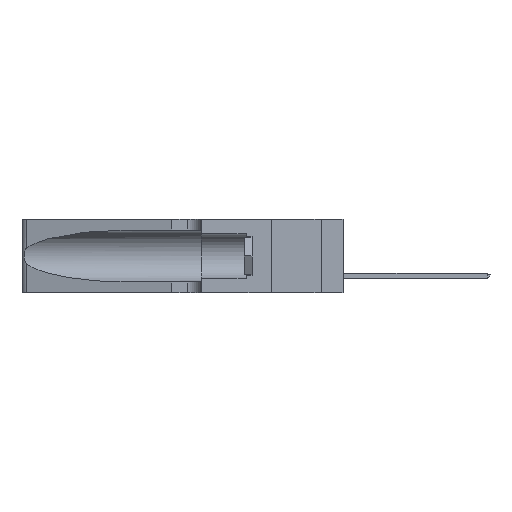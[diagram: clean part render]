
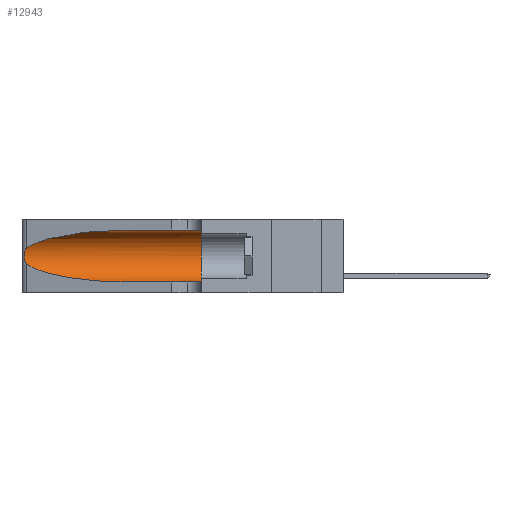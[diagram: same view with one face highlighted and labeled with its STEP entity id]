
A CAD part, left-side view. The second image highlights one B-rep face of the part: STEP entity #12943.
In plain terms, the highlighted cylindrical face has radius 3.308 mm (diameter 6.617 mm), a partial arc.
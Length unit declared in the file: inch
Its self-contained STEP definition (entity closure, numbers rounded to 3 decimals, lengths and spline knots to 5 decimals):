
#659 = LINE ( 'NONE', #36395, #18761 ) ;
#978 = CARTESIAN_POINT ( 'NONE',  ( 0.25487, 1.22718, 0.22369 ) ) ;
#2302 = AXIS2_PLACEMENT_3D ( 'NONE', #22940, #5608, #25963 ) ;
#2400 = VERTEX_POINT ( 'NONE', #12717 ) ;
#2910 = CARTESIAN_POINT ( 'NONE',  ( 0.2373, 1.15595, 0.08982 ) ) ;
#3451 = EDGE_CURVE ( 'NONE', #35282, #16058, #29816, .T. ) ;
#4575 = VERTEX_POINT ( 'NONE', #32277 ) ;
#4591 = ORIENTED_EDGE ( 'NONE', *, *, #21053, .T. ) ;
#4667 = DIRECTION ( 'NONE',  ( 0., 0., -1. ) ) ;
#5193 = EDGE_LOOP ( 'NONE', ( #29478, #30872, #4591, #17342, #19111, #34222 ) ) ;
#5608 = DIRECTION ( 'NONE',  ( 0., 1., 0. ) ) ;
#6177 = CARTESIAN_POINT ( 'NONE',  ( 0.1305, 1.61858, 0.185 ) ) ;
#6301 = CARTESIAN_POINT ( 'NONE',  ( 0.25639, 1.23184, 0.21858 ) ) ;
#6502 = CARTESIAN_POINT ( 'NONE',  ( 0.25487, 1.22718, 0.14631 ) ) ;
#6692 = CARTESIAN_POINT ( 'NONE',  ( 0.25639, 1.23186, 0.15144 ) ) ;
#6892 =( BOUNDED_CURVE ( )  B_SPLINE_CURVE ( 3, ( #6502, #2910, #17912, #18145 ),
 .UNSPECIFIED., .F., .F. ) 
 B_SPLINE_CURVE_WITH_KNOTS ( ( 4, 4 ),
 ( 3.44316, 4.71239 ),
 .UNSPECIFIED. ) 
 CURVE ( )  GEOMETRIC_REPRESENTATION_ITEM ( )  RATIONAL_B_SPLINE_CURVE ( ( 1., 0.87, 0.87, 1. ) ) 
 REPRESENTATION_ITEM ( '' )  );
#7672 = CARTESIAN_POINT ( 'NONE',  ( 0.25487, 1.22718, 0.22369 ) ) ;
#8456 = CIRCLE ( 'NONE', #2302, 0.13025 ) ;
#9170 = CARTESIAN_POINT ( 'NONE',  ( 0.18966, 0.96281, 0.31525 ) ) ;
#9210 = EDGE_CURVE ( 'NONE', #4575, #32043, #659, .T. ) ;
#9219 = CARTESIAN_POINT ( 'NONE',  ( 0.25856, 1.23593, 0.16098 ) ) ;
#9492 = CARTESIAN_POINT ( 'NONE',  ( 0.25555, 1.22993, 0.14849 ) ) ;
#9734 = CARTESIAN_POINT ( 'NONE',  ( 0.26018, 1.23835, 0.19895 ) ) ;
#12605 = CARTESIAN_POINT ( 'NONE',  ( 0.25789, 1.23486, 0.15765 ) ) ;
#12717 = CARTESIAN_POINT ( 'NONE',  ( 0.1305, 0.72297, 0.05475 ) ) ;
#12943 = ADVANCED_FACE ( 'NONE', ( #33346 ), #18430, .F. ) ;
#16058 = VERTEX_POINT ( 'NONE', #29757 ) ;
#17258 = CARTESIAN_POINT ( 'NONE',  ( 0.1305, 1.61858, 0.05475 ) ) ;
#17342 = ORIENTED_EDGE ( 'NONE', *, *, #22458, .T. ) ;
#17370 = VERTEX_POINT ( 'NONE', #20955 ) ;
#17912 = CARTESIAN_POINT ( 'NONE',  ( 0.18966, 0.96281, 0.05475 ) ) ;
#17934 = CARTESIAN_POINT ( 'NONE',  ( 0.25555, 1.22994, 0.2215 ) ) ;
#18028 = EDGE_CURVE ( 'NONE', #32043, #17370, #8456, .T. ) ;
#18145 = CARTESIAN_POINT ( 'NONE',  ( 0.1305, 0.72297, 0.05475 ) ) ;
#18165 = CARTESIAN_POINT ( 'NONE',  ( 0.25854, 1.2359, 0.20912 ) ) ;
#18430 = CYLINDRICAL_SURFACE ( 'NONE', #19570, 0.13025 ) ;
#18761 = VECTOR ( 'NONE', #21990, 39.37008 ) ;
#19111 = ORIENTED_EDGE ( 'NONE', *, *, #18028, .F. ) ;
#19570 = AXIS2_PLACEMENT_3D ( 'NONE', #6177, #21469, #4667 ) ;
#20042 = EDGE_CURVE ( 'NONE', #4575, #35282, #30511, .T. ) ;
#20165 = DIRECTION ( 'NONE',  ( 0., -1., 0. ) ) ;
#20955 = CARTESIAN_POINT ( 'NONE',  ( 0.1305, 0.35, 0.05475 ) ) ;
#21053 = EDGE_CURVE ( 'NONE', #16058, #2400, #6892, .T. ) ;
#21098 = CARTESIAN_POINT ( 'NONE',  ( 0.25487, 1.22718, 0.14631 ) ) ;
#21469 = DIRECTION ( 'NONE',  ( 0., -1., 0. ) ) ;
#21990 = DIRECTION ( 'NONE',  ( 0., -1., 0. ) ) ;
#22344 = CARTESIAN_POINT ( 'NONE',  ( 0.1305, 0.35, 0.31525 ) ) ;
#22458 = EDGE_CURVE ( 'NONE', #2400, #17370, #23091, .T. ) ;
#22940 = CARTESIAN_POINT ( 'NONE',  ( 0.1305, 0.35, 0.185 ) ) ;
#23091 = LINE ( 'NONE', #17258, #28915 ) ;
#23633 = CARTESIAN_POINT ( 'NONE',  ( 0.25487, 1.22718, 0.22369 ) ) ;
#25963 = DIRECTION ( 'NONE',  ( 0., 0., 1. ) ) ;
#26479 = CARTESIAN_POINT ( 'NONE',  ( 0.1305, 0.72297, 0.31525 ) ) ;
#26529 = CARTESIAN_POINT ( 'NONE',  ( 0.26075, 1.23896, 0.19203 ) ) ;
#26603 = CARTESIAN_POINT ( 'NONE',  ( 0.2373, 1.15595, 0.28018 ) ) ;
#28915 = VECTOR ( 'NONE', #20165, 39.37008 ) ;
#29478 = ORIENTED_EDGE ( 'NONE', *, *, #20042, .T. ) ;
#29540 = CARTESIAN_POINT ( 'NONE',  ( 0.25787, 1.23484, 0.2124 ) ) ;
#29757 = CARTESIAN_POINT ( 'NONE',  ( 0.25487, 1.22718, 0.14631 ) ) ;
#29816 = B_SPLINE_CURVE_WITH_KNOTS ( 'NONE', 3,
 ( #23633, #17934, #6301, #29540, #18165, #9734, #26529, #32689, #35605, #9219, #12605, #6692, #9492, #21098 ),
 .UNSPECIFIED., .F., .F.,
 ( 4, 2, 2, 2, 2, 2, 4 ),
 ( 0., 0.00027, 0.00053, 0.00107, 0.0016, 0.00187, 0.00214 ),
 .UNSPECIFIED. ) ;
#30511 =( BOUNDED_CURVE ( )  B_SPLINE_CURVE ( 3, ( #26479, #9170, #26603, #978 ),
 .UNSPECIFIED., .F., .F. ) 
 B_SPLINE_CURVE_WITH_KNOTS ( ( 4, 4 ),
 ( 1.5708, 2.84003 ),
 .UNSPECIFIED. ) 
 CURVE ( )  GEOMETRIC_REPRESENTATION_ITEM ( )  RATIONAL_B_SPLINE_CURVE ( ( 1., 0.87, 0.87, 1. ) ) 
 REPRESENTATION_ITEM ( '' )  );
#30872 = ORIENTED_EDGE ( 'NONE', *, *, #3451, .T. ) ;
#32043 = VERTEX_POINT ( 'NONE', #22344 ) ;
#32277 = CARTESIAN_POINT ( 'NONE',  ( 0.1305, 0.72297, 0.31525 ) ) ;
#32689 = CARTESIAN_POINT ( 'NONE',  ( 0.26075, 1.23896, 0.178 ) ) ;
#33346 = FACE_OUTER_BOUND ( 'NONE', #5193, .T. ) ;
#34222 = ORIENTED_EDGE ( 'NONE', *, *, #9210, .F. ) ;
#35282 = VERTEX_POINT ( 'NONE', #7672 ) ;
#35605 = CARTESIAN_POINT ( 'NONE',  ( 0.26017, 1.23833, 0.17102 ) ) ;
#36395 = CARTESIAN_POINT ( 'NONE',  ( 0.1305, 1.61858, 0.31525 ) ) ;
